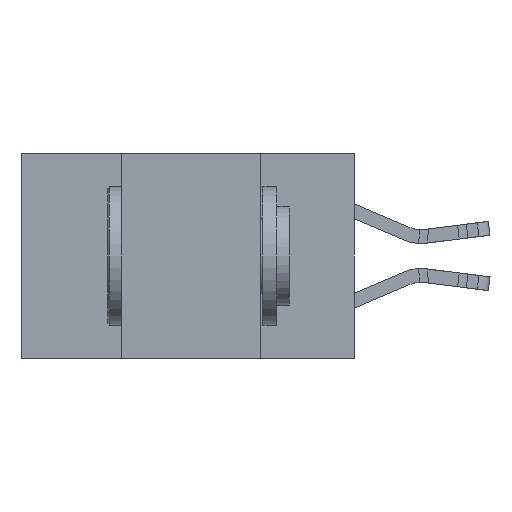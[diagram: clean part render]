
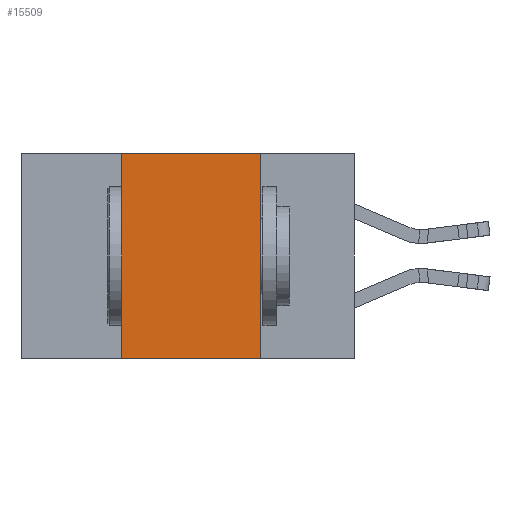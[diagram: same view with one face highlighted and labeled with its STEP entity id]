
A CAD part, left-side view. The second image highlights one B-rep face of the part: STEP entity #15509.
In plain terms, the highlighted planar face has unit normal (-1, 0, 0).
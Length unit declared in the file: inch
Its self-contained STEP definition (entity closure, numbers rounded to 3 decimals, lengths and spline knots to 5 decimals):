
#1740 = EDGE_CURVE ( 'NONE', #26537, #23864, #12897, .T. ) ;
#3706 = PLANE ( 'NONE',  #12857 ) ;
#4389 = CARTESIAN_POINT ( 'NONE',  ( 0., 0.17, -0.37 ) ) ;
#4443 = VECTOR ( 'NONE', #23936, 39.37008 ) ;
#5155 = LINE ( 'NONE', #28329, #4443 ) ;
#6261 = CARTESIAN_POINT ( 'NONE',  ( 0., 0.42, -0.37 ) ) ;
#6406 = FACE_OUTER_BOUND ( 'NONE', #20360, .T. ) ;
#6519 = LINE ( 'NONE', #6910, #25564 ) ;
#6751 = VECTOR ( 'NONE', #21663, 39.37008 ) ;
#6910 = CARTESIAN_POINT ( 'NONE',  ( 0., 0.6, 0. ) ) ;
#7659 = VECTOR ( 'NONE', #21126, 39.37008 ) ;
#8217 = CARTESIAN_POINT ( 'NONE',  ( 0., 0.6, 0. ) ) ;
#8263 = ORIENTED_EDGE ( 'NONE', *, *, #1740, .F. ) ;
#8388 = CARTESIAN_POINT ( 'NONE',  ( 0., 0.42, -0.37 ) ) ;
#9357 = VERTEX_POINT ( 'NONE', #18508 ) ;
#10395 = VERTEX_POINT ( 'NONE', #8388 ) ;
#10450 = DIRECTION ( 'NONE',  ( 0., 0., -1. ) ) ;
#12857 = AXIS2_PLACEMENT_3D ( 'NONE', #8217, #23705, #10450 ) ;
#12897 = LINE ( 'NONE', #21792, #7659 ) ;
#14172 = ORIENTED_EDGE ( 'NONE', *, *, #24569, .F. ) ;
#14774 = EDGE_CURVE ( 'NONE', #10395, #23864, #5155, .T. ) ;
#15509 = ADVANCED_FACE ( 'NONE', ( #6406 ), #3706, .F. ) ;
#18508 = CARTESIAN_POINT ( 'NONE',  ( 0., 0.42, 0. ) ) ;
#20360 = EDGE_LOOP ( 'NONE', ( #8263, #14172, #21425, #22814 ) ) ;
#21126 = DIRECTION ( 'NONE',  ( 0., 0., -1. ) ) ;
#21425 = ORIENTED_EDGE ( 'NONE', *, *, #26598, .F. ) ;
#21663 = DIRECTION ( 'NONE',  ( 0., 0., 1. ) ) ;
#21792 = CARTESIAN_POINT ( 'NONE',  ( 0., 0.17, -0.37 ) ) ;
#22407 = DIRECTION ( 'NONE',  ( 0., -1., 0. ) ) ;
#22814 = ORIENTED_EDGE ( 'NONE', *, *, #14774, .T. ) ;
#23705 = DIRECTION ( 'NONE',  ( 1., 0., 0. ) ) ;
#23864 = VERTEX_POINT ( 'NONE', #4389 ) ;
#23936 = DIRECTION ( 'NONE',  ( 0., -1., 0. ) ) ;
#24388 = LINE ( 'NONE', #6261, #6751 ) ;
#24569 = EDGE_CURVE ( 'NONE', #9357, #26537, #6519, .T. ) ;
#25564 = VECTOR ( 'NONE', #22407, 39.37008 ) ;
#26537 = VERTEX_POINT ( 'NONE', #28092 ) ;
#26598 = EDGE_CURVE ( 'NONE', #10395, #9357, #24388, .T. ) ;
#28092 = CARTESIAN_POINT ( 'NONE',  ( 0., 0.17, 0. ) ) ;
#28329 = CARTESIAN_POINT ( 'NONE',  ( 0., 0.6, -0.37 ) ) ;
